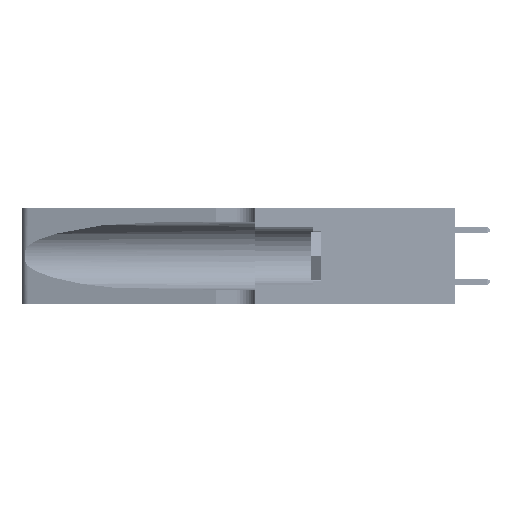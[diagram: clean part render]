
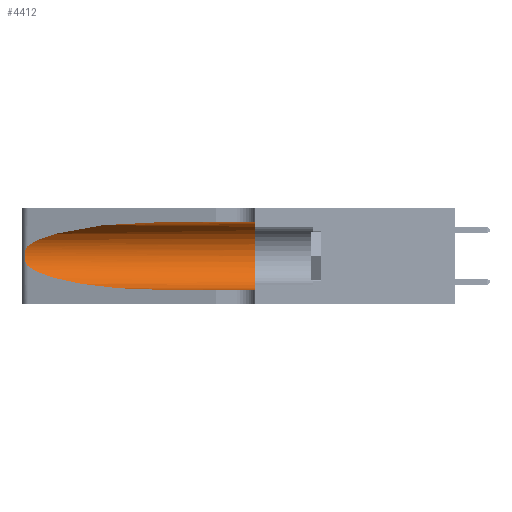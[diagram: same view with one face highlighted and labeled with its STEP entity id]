
A CAD part, left-side view. The second image highlights one B-rep face of the part: STEP entity #4412.
In plain terms, the highlighted cylindrical face has radius 3.308 mm (diameter 6.617 mm), a partial arc.
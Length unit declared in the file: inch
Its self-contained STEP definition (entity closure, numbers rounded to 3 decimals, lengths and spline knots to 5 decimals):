
#1518 = CARTESIAN_POINT ( 'NONE',  ( 0.25639, 1.23184, 0.21858 ) ) ;
#1973 = CARTESIAN_POINT ( 'NONE',  ( 0.18966, 0.96281, 0.31525 ) ) ;
#2643 = AXIS2_PLACEMENT_3D ( 'NONE', #26180, #22019, #25472 ) ;
#2749 = CARTESIAN_POINT ( 'NONE',  ( 0.1305, 0.72297, 0.05475 ) ) ;
#2771 = CARTESIAN_POINT ( 'NONE',  ( 0.18966, 0.96281, 0.05475 ) ) ;
#4412 = ADVANCED_FACE ( 'NONE', ( #49677 ), #48398, .F. ) ;
#4750 = CARTESIAN_POINT ( 'NONE',  ( 0.25487, 1.22718, 0.22369 ) ) ;
#4784 = ORIENTED_EDGE ( 'NONE', *, *, #17981, .T. ) ;
#5554 = DIRECTION ( 'NONE',  ( 0., -1., 0. ) ) ;
#5660 = CARTESIAN_POINT ( 'NONE',  ( 0.26017, 1.23833, 0.17102 ) ) ;
#6023 = CARTESIAN_POINT ( 'NONE',  ( 0.25487, 1.22718, 0.22369 ) ) ;
#6553 = DIRECTION ( 'NONE',  ( 0., 0., 1. ) ) ;
#6998 = EDGE_CURVE ( 'NONE', #52758, #16296, #42434, .T. ) ;
#7127 = AXIS2_PLACEMENT_3D ( 'NONE', #18669, #39472, #6553 ) ;
#10082 = CARTESIAN_POINT ( 'NONE',  ( 0.1305, 1.61858, 0.31525 ) ) ;
#10181 = CARTESIAN_POINT ( 'NONE',  ( 0.25789, 1.23486, 0.15765 ) ) ;
#11285 = VERTEX_POINT ( 'NONE', #4750 ) ;
#12254 = EDGE_CURVE ( 'NONE', #32897, #18924, #17221, .T. ) ;
#13024 = ORIENTED_EDGE ( 'NONE', *, *, #6998, .T. ) ;
#13149 = CARTESIAN_POINT ( 'NONE',  ( 0.1305, 0.35, 0.05475 ) ) ;
#14534 = CARTESIAN_POINT ( 'NONE',  ( 0.26075, 1.23896, 0.19203 ) ) ;
#14965 = DIRECTION ( 'NONE',  ( 0., -1., 0. ) ) ;
#15171 = CARTESIAN_POINT ( 'NONE',  ( 0.2373, 1.15595, 0.28018 ) ) ;
#16170 = VECTOR ( 'NONE', #14965, 39.37008 ) ;
#16296 = VERTEX_POINT ( 'NONE', #2749 ) ;
#16546 = VECTOR ( 'NONE', #5554, 39.37008 ) ;
#17221 = LINE ( 'NONE', #10082, #16546 ) ;
#17618 = CARTESIAN_POINT ( 'NONE',  ( 0.1305, 0.72297, 0.31525 ) ) ;
#17981 = EDGE_CURVE ( 'NONE', #32897, #11285, #22212, .T. ) ;
#18669 = CARTESIAN_POINT ( 'NONE',  ( 0.1305, 0.35, 0.185 ) ) ;
#18924 = VERTEX_POINT ( 'NONE', #41832 ) ;
#19679 = CARTESIAN_POINT ( 'NONE',  ( 0.1305, 0.72297, 0.05475 ) ) ;
#22019 = DIRECTION ( 'NONE',  ( 0., -1., 0. ) ) ;
#22212 =( BOUNDED_CURVE ( )  B_SPLINE_CURVE ( 3, ( #35417, #1973, #15171, #48392 ),
 .UNSPECIFIED., .F., .F. ) 
 B_SPLINE_CURVE_WITH_KNOTS ( ( 4, 4 ),
 ( 1.5708, 2.84003 ),
 .UNSPECIFIED. ) 
 CURVE ( )  GEOMETRIC_REPRESENTATION_ITEM ( )  RATIONAL_B_SPLINE_CURVE ( ( 1., 0.87, 0.87, 1. ) ) 
 REPRESENTATION_ITEM ( '' )  );
#25251 = EDGE_CURVE ( 'NONE', #18924, #27945, #31581, .T. ) ;
#25472 = DIRECTION ( 'NONE',  ( 0., 0., -1. ) ) ;
#26180 = CARTESIAN_POINT ( 'NONE',  ( 0.1305, 1.61858, 0.185 ) ) ;
#27945 = VERTEX_POINT ( 'NONE', #13149 ) ;
#28047 = CARTESIAN_POINT ( 'NONE',  ( 0.2373, 1.15595, 0.08982 ) ) ;
#29824 = ORIENTED_EDGE ( 'NONE', *, *, #25251, .F. ) ;
#29833 = ORIENTED_EDGE ( 'NONE', *, *, #43525, .T. ) ;
#30153 = EDGE_LOOP ( 'NONE', ( #4784, #44416, #13024, #29833, #29824, #30545 ) ) ;
#30406 = CARTESIAN_POINT ( 'NONE',  ( 0.25787, 1.23484, 0.2124 ) ) ;
#30545 = ORIENTED_EDGE ( 'NONE', *, *, #12254, .F. ) ;
#30693 = CARTESIAN_POINT ( 'NONE',  ( 0.25487, 1.22718, 0.14631 ) ) ;
#31581 = CIRCLE ( 'NONE', #7127, 0.13025 ) ;
#32897 = VERTEX_POINT ( 'NONE', #17618 ) ;
#34939 = CARTESIAN_POINT ( 'NONE',  ( 0.25854, 1.2359, 0.20912 ) ) ;
#35132 = CARTESIAN_POINT ( 'NONE',  ( 0.26018, 1.23835, 0.19895 ) ) ;
#35417 = CARTESIAN_POINT ( 'NONE',  ( 0.1305, 0.72297, 0.31525 ) ) ;
#38150 = LINE ( 'NONE', #48018, #16170 ) ;
#38755 = CARTESIAN_POINT ( 'NONE',  ( 0.25856, 1.23593, 0.16098 ) ) ;
#39111 = CARTESIAN_POINT ( 'NONE',  ( 0.25487, 1.22718, 0.14631 ) ) ;
#39472 = DIRECTION ( 'NONE',  ( 0., 1., 0. ) ) ;
#39663 = EDGE_CURVE ( 'NONE', #11285, #52758, #45365, .T. ) ;
#41832 = CARTESIAN_POINT ( 'NONE',  ( 0.1305, 0.35, 0.31525 ) ) ;
#42434 =( BOUNDED_CURVE ( )  B_SPLINE_CURVE ( 3, ( #39111, #28047, #2771, #19679 ),
 .UNSPECIFIED., .F., .F. ) 
 B_SPLINE_CURVE_WITH_KNOTS ( ( 4, 4 ),
 ( 3.44316, 4.71239 ),
 .UNSPECIFIED. ) 
 CURVE ( )  GEOMETRIC_REPRESENTATION_ITEM ( )  RATIONAL_B_SPLINE_CURVE ( ( 1., 0.87, 0.87, 1. ) ) 
 REPRESENTATION_ITEM ( '' )  );
#43087 = CARTESIAN_POINT ( 'NONE',  ( 0.25555, 1.22994, 0.2215 ) ) ;
#43525 = EDGE_CURVE ( 'NONE', #16296, #27945, #38150, .T. ) ;
#44416 = ORIENTED_EDGE ( 'NONE', *, *, #39663, .T. ) ;
#45365 = B_SPLINE_CURVE_WITH_KNOTS ( 'NONE', 3,
 ( #6023, #43087, #1518, #30406, #34939, #35132, #14534, #47385, #5660, #38755, #10181, #47021, #51150, #51533 ),
 .UNSPECIFIED., .F., .F.,
 ( 4, 2, 2, 2, 2, 2, 4 ),
 ( 0., 0.00027, 0.00053, 0.00107, 0.0016, 0.00187, 0.00214 ),
 .UNSPECIFIED. ) ;
#47021 = CARTESIAN_POINT ( 'NONE',  ( 0.25639, 1.23186, 0.15144 ) ) ;
#47385 = CARTESIAN_POINT ( 'NONE',  ( 0.26075, 1.23896, 0.178 ) ) ;
#48018 = CARTESIAN_POINT ( 'NONE',  ( 0.1305, 1.61858, 0.05475 ) ) ;
#48392 = CARTESIAN_POINT ( 'NONE',  ( 0.25487, 1.22718, 0.22369 ) ) ;
#48398 = CYLINDRICAL_SURFACE ( 'NONE', #2643, 0.13025 ) ;
#49677 = FACE_OUTER_BOUND ( 'NONE', #30153, .T. ) ;
#51150 = CARTESIAN_POINT ( 'NONE',  ( 0.25555, 1.22993, 0.14849 ) ) ;
#51533 = CARTESIAN_POINT ( 'NONE',  ( 0.25487, 1.22718, 0.14631 ) ) ;
#52758 = VERTEX_POINT ( 'NONE', #30693 ) ;
